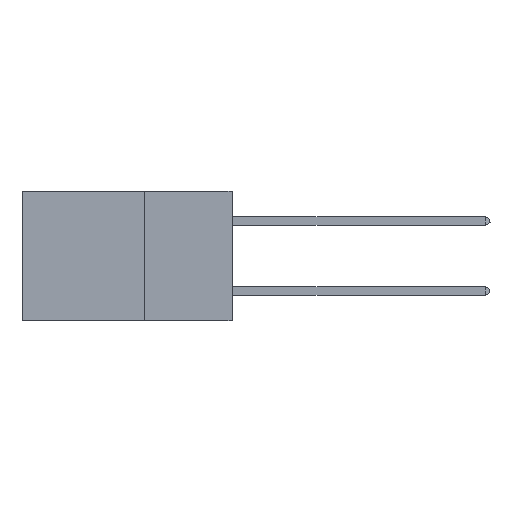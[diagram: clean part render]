
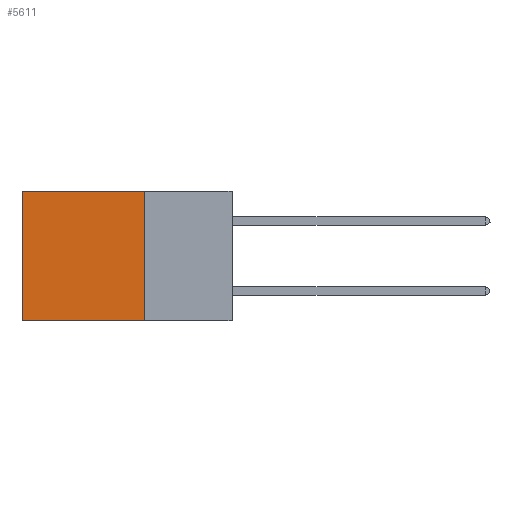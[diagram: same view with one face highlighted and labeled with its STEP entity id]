
A CAD part, left-side view. The second image highlights one B-rep face of the part: STEP entity #5611.
In plain terms, the highlighted planar face has unit normal (-1, 0, 0).
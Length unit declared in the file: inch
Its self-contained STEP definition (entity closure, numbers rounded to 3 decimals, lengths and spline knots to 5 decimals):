
#187 = DIRECTION ( 'NONE',  ( 0., 0., -1. ) ) ;
#460 = VERTEX_POINT ( 'NONE', #4096 ) ;
#2193 = DIRECTION ( 'NONE',  ( 0., 1., 0. ) ) ;
#2202 = DIRECTION ( 'NONE',  ( 0., 0., -1. ) ) ;
#2274 = LINE ( 'NONE', #12820, #12432 ) ;
#2607 = AXIS2_PLACEMENT_3D ( 'NONE', #3120, #11437, #2202 ) ;
#3006 = EDGE_CURVE ( 'NONE', #3072, #13207, #11753, .T. ) ;
#3072 = VERTEX_POINT ( 'NONE', #14358 ) ;
#3120 = CARTESIAN_POINT ( 'NONE',  ( 0.2875, 0.25, 0. ) ) ;
#3242 = EDGE_CURVE ( 'NONE', #5178, #460, #2274, .T. ) ;
#4096 = CARTESIAN_POINT ( 'NONE',  ( 0.2875, 0.6, 0. ) ) ;
#4424 = VECTOR ( 'NONE', #4974, 39.37008 ) ;
#4765 = ORIENTED_EDGE ( 'NONE', *, *, #10615, .T. ) ;
#4974 = DIRECTION ( 'NONE',  ( 0., 1., 0. ) ) ;
#5178 = VERTEX_POINT ( 'NONE', #14623 ) ;
#5506 = FACE_OUTER_BOUND ( 'NONE', #15028, .T. ) ;
#5535 = LINE ( 'NONE', #5840, #12058 ) ;
#5611 = ADVANCED_FACE ( 'NONE', ( #5506 ), #11513, .F. ) ;
#5840 = CARTESIAN_POINT ( 'NONE',  ( 0.2875, 0.25, 0. ) ) ;
#7117 = CARTESIAN_POINT ( 'NONE',  ( 0.2875, 0.6, 0. ) ) ;
#7993 = ORIENTED_EDGE ( 'NONE', *, *, #12125, .F. ) ;
#8441 = ORIENTED_EDGE ( 'NONE', *, *, #3006, .F. ) ;
#8851 = VECTOR ( 'NONE', #187, 39.37008 ) ;
#10004 = ORIENTED_EDGE ( 'NONE', *, *, #3242, .T. ) ;
#10153 = CARTESIAN_POINT ( 'NONE',  ( 0.2875, 0.6, -0.37 ) ) ;
#10531 = DIRECTION ( 'NONE',  ( 0., 0., -1. ) ) ;
#10615 = EDGE_CURVE ( 'NONE', #460, #13207, #13975, .T. ) ;
#11437 = DIRECTION ( 'NONE',  ( 1., 0., 0. ) ) ;
#11513 = PLANE ( 'NONE',  #2607 ) ;
#11753 = LINE ( 'NONE', #14429, #4424 ) ;
#12058 = VECTOR ( 'NONE', #10531, 39.37008 ) ;
#12125 = EDGE_CURVE ( 'NONE', #5178, #3072, #5535, .T. ) ;
#12432 = VECTOR ( 'NONE', #2193, 39.37008 ) ;
#12820 = CARTESIAN_POINT ( 'NONE',  ( 0.2875, 0.25, 0. ) ) ;
#13207 = VERTEX_POINT ( 'NONE', #10153 ) ;
#13975 = LINE ( 'NONE', #7117, #8851 ) ;
#14358 = CARTESIAN_POINT ( 'NONE',  ( 0.2875, 0.25, -0.37 ) ) ;
#14429 = CARTESIAN_POINT ( 'NONE',  ( 0.2875, 0.25, -0.37 ) ) ;
#14623 = CARTESIAN_POINT ( 'NONE',  ( 0.2875, 0.25, 0. ) ) ;
#15028 = EDGE_LOOP ( 'NONE', ( #4765, #8441, #7993, #10004 ) ) ;
